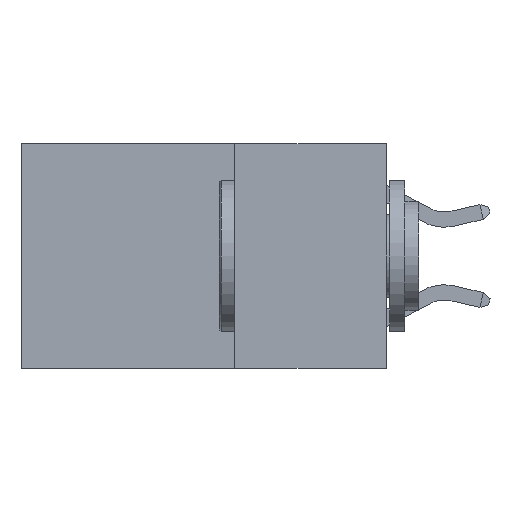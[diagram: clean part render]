
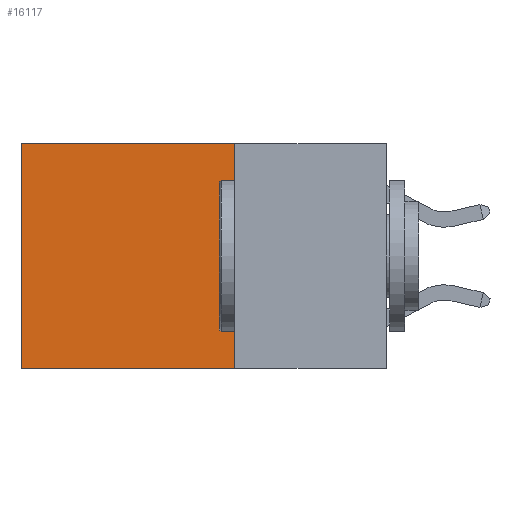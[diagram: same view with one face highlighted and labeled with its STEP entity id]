
A CAD part, left-side view. The second image highlights one B-rep face of the part: STEP entity #16117.
In plain terms, the highlighted planar face has unit normal (-1, 0, 0).
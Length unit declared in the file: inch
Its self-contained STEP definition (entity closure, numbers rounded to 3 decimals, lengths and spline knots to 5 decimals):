
#821 = ORIENTED_EDGE ( 'NONE', *, *, #9884, .F. ) ;
#1451 = VERTEX_POINT ( 'NONE', #17312 ) ;
#1853 = VECTOR ( 'NONE', #15105, 39.37008 ) ;
#2044 = VECTOR ( 'NONE', #16414, 39.37008 ) ;
#2535 = CARTESIAN_POINT ( 'NONE',  ( 0.2625, 0.25, -0.37 ) ) ;
#2927 = CARTESIAN_POINT ( 'NONE',  ( 0.2625, 0.25, 0. ) ) ;
#2958 = VECTOR ( 'NONE', #15568, 39.37008 ) ;
#3444 = VERTEX_POINT ( 'NONE', #15482 ) ;
#5371 = DIRECTION ( 'NONE',  ( 0., 0., -1. ) ) ;
#5895 = CARTESIAN_POINT ( 'NONE',  ( 0.2625, 0.6, -0.37 ) ) ;
#6155 = ORIENTED_EDGE ( 'NONE', *, *, #7745, .F. ) ;
#7221 = LINE ( 'NONE', #2535, #2044 ) ;
#7745 = EDGE_CURVE ( 'NONE', #1451, #14345, #19660, .T. ) ;
#8683 = AXIS2_PLACEMENT_3D ( 'NONE', #14773, #19339, #5371 ) ;
#8809 = CARTESIAN_POINT ( 'NONE',  ( 0.2625, 0.25, 0. ) ) ;
#8860 = ORIENTED_EDGE ( 'NONE', *, *, #16955, .T. ) ;
#8932 = CARTESIAN_POINT ( 'NONE',  ( 0.2625, 0.25, -0.37 ) ) ;
#9884 = EDGE_CURVE ( 'NONE', #14345, #11590, #7221, .T. ) ;
#10567 = EDGE_CURVE ( 'NONE', #1451, #3444, #17117, .T. ) ;
#11590 = VERTEX_POINT ( 'NONE', #5895 ) ;
#12602 = LINE ( 'NONE', #15799, #14094 ) ;
#13041 = FACE_OUTER_BOUND ( 'NONE', #18803, .T. ) ;
#13235 = PLANE ( 'NONE',  #8683 ) ;
#14094 = VECTOR ( 'NONE', #17251, 39.37008 ) ;
#14345 = VERTEX_POINT ( 'NONE', #8932 ) ;
#14773 = CARTESIAN_POINT ( 'NONE',  ( 0.2625, 0.25, 0. ) ) ;
#15105 = DIRECTION ( 'NONE',  ( 0., 0., -1. ) ) ;
#15482 = CARTESIAN_POINT ( 'NONE',  ( 0.2625, 0.6, 0. ) ) ;
#15568 = DIRECTION ( 'NONE',  ( 0., 1., 0. ) ) ;
#15799 = CARTESIAN_POINT ( 'NONE',  ( 0.2625, 0.6, 0. ) ) ;
#16117 = ADVANCED_FACE ( 'NONE', ( #13041 ), #13235, .F. ) ;
#16350 = ORIENTED_EDGE ( 'NONE', *, *, #10567, .T. ) ;
#16414 = DIRECTION ( 'NONE',  ( 0., 1., 0. ) ) ;
#16955 = EDGE_CURVE ( 'NONE', #3444, #11590, #12602, .T. ) ;
#17117 = LINE ( 'NONE', #2927, #2958 ) ;
#17251 = DIRECTION ( 'NONE',  ( 0., 0., -1. ) ) ;
#17312 = CARTESIAN_POINT ( 'NONE',  ( 0.2625, 0.25, 0. ) ) ;
#18803 = EDGE_LOOP ( 'NONE', ( #8860, #821, #6155, #16350 ) ) ;
#19339 = DIRECTION ( 'NONE',  ( 1., 0., 0. ) ) ;
#19660 = LINE ( 'NONE', #8809, #1853 ) ;
